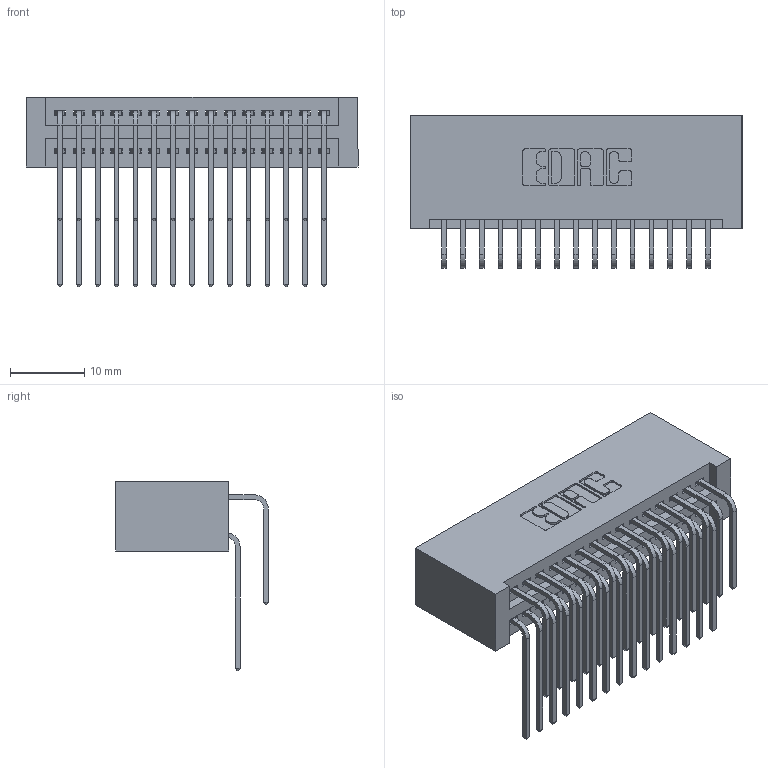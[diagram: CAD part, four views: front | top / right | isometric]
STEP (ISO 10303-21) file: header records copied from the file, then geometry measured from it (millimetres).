
FILE_DESCRIPTION (( 'STEP AP203' ), '1' );
FILE_NAME ('345-030-559-201.STEP', '2019-10-28T02:50:36', ( '' ), ( '' ), 'SwSTEP 2.0', 'SolidWorks 2016', '' );
FILE_SCHEMA (( 'CONFIG_CONTROL_DESIGN' ));
Length unit declared in the file: inch
Products named in the file (4): 345-030-559-201; 345-292-001_558 559 Tail - 1; 345-292-001_559 Tail - 2; 345 Part_No Mounting Lugs
Assembly tree (31 placements, depth 2):
  345-030-559-201
    345 Part_No Mounting Lugs
    345-292-001_558 559 Tail - 1  x15
    345-292-001_559 Tail - 2  x15
Bounding box: 44.7 x 20.56 x 25.53 mm (x, y, z)
Volume: 4880.9 mm3; surface area: 7809 mm2
Topology: 31 solids, 31 shells, 1678 faces, 4967 edges, 3270 vertices
Faces by surface type: plane 1126, cylinder 552
Entity records: 16779 total; most frequent: CARTESIAN_POINT 2883, ORIENTED_EDGE 2766, DIRECTION 2543, EDGE_CURVE 1383, LINE 1159, VECTOR 1159, VERTEX_POINT 918, AXIS2_PLACEMENT_3D 692
